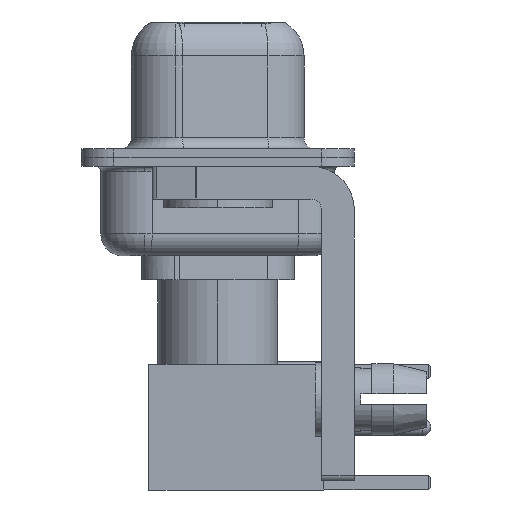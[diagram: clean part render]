
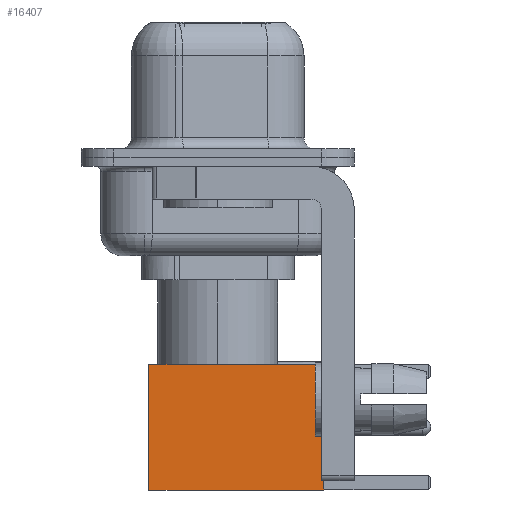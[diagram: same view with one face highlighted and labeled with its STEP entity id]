
A CAD part, left-side view. The second image highlights one B-rep face of the part: STEP entity #16407.
In plain terms, the highlighted face is planar.
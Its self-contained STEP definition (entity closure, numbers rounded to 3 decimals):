
#145 = PLANE ( 'NONE',  #2929 ) ;
#675 = VECTOR ( 'NONE', #23838, 1000. ) ;
#1072 = EDGE_CURVE ( 'NONE', #13956, #2113, #24090, .T. ) ;
#1259 = CARTESIAN_POINT ( 'NONE',  ( 2.875, 2.875, 0. ) ) ;
#2113 = VERTEX_POINT ( 'NONE', #13313 ) ;
#2647 = LINE ( 'NONE', #10654, #24660 ) ;
#2929 = AXIS2_PLACEMENT_3D ( 'NONE', #23030, #19084, #18958 ) ;
#3041 = DIRECTION ( 'NONE',  ( 0., 0., -1. ) ) ;
#4642 = VECTOR ( 'NONE', #5606, 1000. ) ;
#4861 = VERTEX_POINT ( 'NONE', #10319 ) ;
#5606 = DIRECTION ( 'NONE',  ( 0., 0., -1. ) ) ;
#5947 = VERTEX_POINT ( 'NONE', #19785 ) ;
#6500 = CARTESIAN_POINT ( 'NONE',  ( 2.875, 2.875, 8. ) ) ;
#7340 = ORIENTED_EDGE ( 'NONE', *, *, #1072, .F. ) ;
#7403 = ORIENTED_EDGE ( 'NONE', *, *, #21062, .F. ) ;
#7543 = FACE_OUTER_BOUND ( 'NONE', #14331, .T. ) ;
#8031 = VECTOR ( 'NONE', #3041, 1000. ) ;
#8065 = ORIENTED_EDGE ( 'NONE', *, *, #10139, .T. ) ;
#9167 = CARTESIAN_POINT ( 'NONE',  ( -2.875, 2.875, 0. ) ) ;
#9208 = ORIENTED_EDGE ( 'NONE', *, *, #10462, .T. ) ;
#10139 = EDGE_CURVE ( 'NONE', #4861, #5947, #2647, .T. ) ;
#10319 = CARTESIAN_POINT ( 'NONE',  ( 2.875, 2.875, 0. ) ) ;
#10462 = EDGE_CURVE ( 'NONE', #13956, #4861, #20566, .T. ) ;
#10654 = CARTESIAN_POINT ( 'NONE',  ( 0., 2.875, 0. ) ) ;
#13313 = CARTESIAN_POINT ( 'NONE',  ( -2.875, 2.875, 8. ) ) ;
#13956 = VERTEX_POINT ( 'NONE', #6500 ) ;
#14331 = EDGE_LOOP ( 'NONE', ( #9208, #8065, #7403, #7340 ) ) ;
#14341 = DIRECTION ( 'NONE',  ( -1., 0., 0. ) ) ;
#14411 = CARTESIAN_POINT ( 'NONE',  ( 0., 2.875, 8. ) ) ;
#15253 = LINE ( 'NONE', #9167, #4642 ) ;
#16407 = ADVANCED_FACE ( 'NONE', ( #7543 ), #145, .T. ) ;
#18958 = DIRECTION ( 'NONE',  ( 0., 0., 1. ) ) ;
#19084 = DIRECTION ( 'NONE',  ( 0., 1., 0. ) ) ;
#19785 = CARTESIAN_POINT ( 'NONE',  ( -2.875, 2.875, 0. ) ) ;
#20566 = LINE ( 'NONE', #1259, #8031 ) ;
#21062 = EDGE_CURVE ( 'NONE', #2113, #5947, #15253, .T. ) ;
#23030 = CARTESIAN_POINT ( 'NONE',  ( 2.875, 2.875, 0. ) ) ;
#23838 = DIRECTION ( 'NONE',  ( -1., 0., 0. ) ) ;
#24090 = LINE ( 'NONE', #14411, #675 ) ;
#24660 = VECTOR ( 'NONE', #14341, 1000. ) ;
